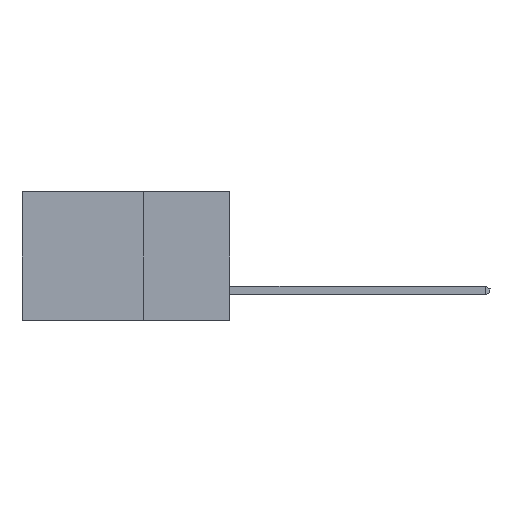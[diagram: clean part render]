
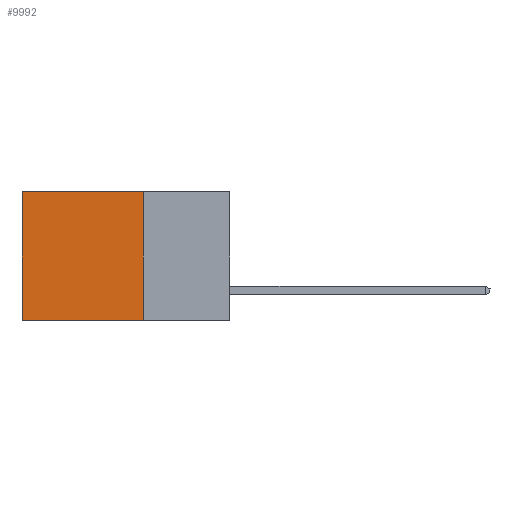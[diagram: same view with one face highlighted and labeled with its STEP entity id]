
A CAD part, left-side view. The second image highlights one B-rep face of the part: STEP entity #9992.
In plain terms, the highlighted planar face has unit normal (-1, 0, 0).
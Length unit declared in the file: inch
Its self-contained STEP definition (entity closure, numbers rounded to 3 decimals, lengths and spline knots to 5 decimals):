
#47 = CARTESIAN_POINT ( 'NONE',  ( 0.2615, 0.25, -0.37 ) ) ;
#856 = LINE ( 'NONE', #6132, #5031 ) ;
#970 = CARTESIAN_POINT ( 'NONE',  ( 0.2615, 0.6, -0.37 ) ) ;
#2079 = AXIS2_PLACEMENT_3D ( 'NONE', #47, #11133, #9025 ) ;
#2204 = CARTESIAN_POINT ( 'NONE',  ( 0.2615, 0.25, 0. ) ) ;
#3392 = EDGE_CURVE ( 'NONE', #9221, #9614, #8552, .T. ) ;
#3396 = CARTESIAN_POINT ( 'NONE',  ( 0.2615, 0.6, -0.37 ) ) ;
#3484 = FACE_OUTER_BOUND ( 'NONE', #10491, .T. ) ;
#3614 = LINE ( 'NONE', #3396, #13441 ) ;
#4020 = EDGE_CURVE ( 'NONE', #9614, #8426, #856, .T. ) ;
#4340 = CARTESIAN_POINT ( 'NONE',  ( 0.2615, 0.25, 0. ) ) ;
#4435 = PLANE ( 'NONE',  #2079 ) ;
#5031 = VECTOR ( 'NONE', #11013, 39.37008 ) ;
#5647 = CARTESIAN_POINT ( 'NONE',  ( 0.2615, 0.25, -0.37 ) ) ;
#6132 = CARTESIAN_POINT ( 'NONE',  ( 0.2615, 0.25, -0.37 ) ) ;
#7262 = EDGE_CURVE ( 'NONE', #14213, #8426, #3614, .T. ) ;
#7823 = CARTESIAN_POINT ( 'NONE',  ( 0.2615, 0.6, 0. ) ) ;
#8426 = VERTEX_POINT ( 'NONE', #970 ) ;
#8481 = CARTESIAN_POINT ( 'NONE',  ( 0.2615, 0.25, -0.37 ) ) ;
#8552 = LINE ( 'NONE', #8481, #9213 ) ;
#9025 = DIRECTION ( 'NONE',  ( 0., 0., -1. ) ) ;
#9061 = DIRECTION ( 'NONE',  ( 0., 1., 0. ) ) ;
#9213 = VECTOR ( 'NONE', #12993, 39.37008 ) ;
#9221 = VERTEX_POINT ( 'NONE', #4340 ) ;
#9552 = EDGE_CURVE ( 'NONE', #9221, #14213, #12047, .T. ) ;
#9614 = VERTEX_POINT ( 'NONE', #5647 ) ;
#9992 = ADVANCED_FACE ( 'NONE', ( #3484 ), #4435, .F. ) ;
#10491 = EDGE_LOOP ( 'NONE', ( #11545, #14115, #13265, #13699 ) ) ;
#11013 = DIRECTION ( 'NONE',  ( 0., 1., 0. ) ) ;
#11133 = DIRECTION ( 'NONE',  ( 1., 0., 0. ) ) ;
#11333 = DIRECTION ( 'NONE',  ( 0., 0., -1. ) ) ;
#11545 = ORIENTED_EDGE ( 'NONE', *, *, #7262, .T. ) ;
#12047 = LINE ( 'NONE', #2204, #14175 ) ;
#12993 = DIRECTION ( 'NONE',  ( 0., 0., -1. ) ) ;
#13265 = ORIENTED_EDGE ( 'NONE', *, *, #3392, .F. ) ;
#13441 = VECTOR ( 'NONE', #11333, 39.37008 ) ;
#13699 = ORIENTED_EDGE ( 'NONE', *, *, #9552, .T. ) ;
#14115 = ORIENTED_EDGE ( 'NONE', *, *, #4020, .F. ) ;
#14175 = VECTOR ( 'NONE', #9061, 39.37008 ) ;
#14213 = VERTEX_POINT ( 'NONE', #7823 ) ;
